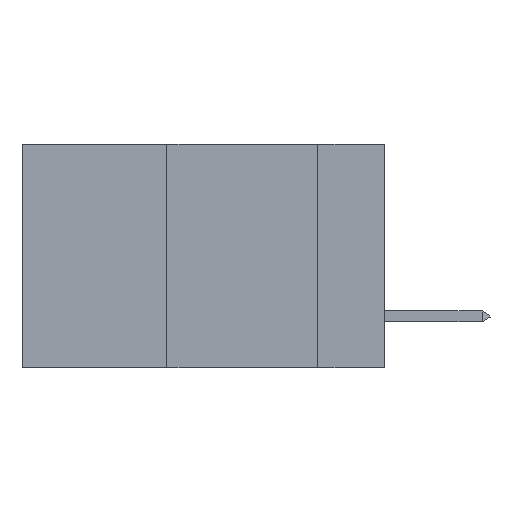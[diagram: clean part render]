
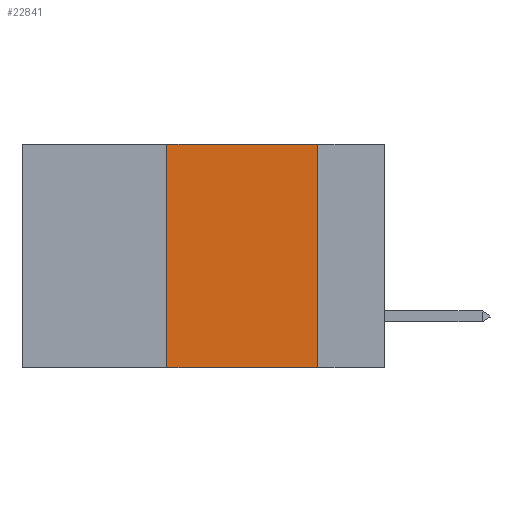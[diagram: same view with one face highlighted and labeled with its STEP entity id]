
A CAD part, left-side view. The second image highlights one B-rep face of the part: STEP entity #22841.
In plain terms, the highlighted planar face has unit normal (-1, 0, 0).
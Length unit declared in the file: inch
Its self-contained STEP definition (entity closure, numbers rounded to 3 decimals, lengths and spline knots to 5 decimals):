
#185 = CARTESIAN_POINT ( 'NONE',  ( 0., 0.6, 0. ) ) ;
#792 = CARTESIAN_POINT ( 'NONE',  ( 0., 0.36, 0. ) ) ;
#1187 = VERTEX_POINT ( 'NONE', #9490 ) ;
#1258 = VECTOR ( 'NONE', #18300, 39.37008 ) ;
#2068 = CARTESIAN_POINT ( 'NONE',  ( 0., 0.11, 0. ) ) ;
#2605 = DIRECTION ( 'NONE',  ( 0., 0., -1. ) ) ;
#3357 = ORIENTED_EDGE ( 'NONE', *, *, #15038, .T. ) ;
#3580 = ORIENTED_EDGE ( 'NONE', *, *, #14342, .F. ) ;
#4287 = DIRECTION ( 'NONE',  ( 1., 0., 0. ) ) ;
#4668 = CARTESIAN_POINT ( 'NONE',  ( 0., 0.11, -0.37 ) ) ;
#5337 = EDGE_CURVE ( 'NONE', #1187, #9684, #16919, .T. ) ;
#5397 = DIRECTION ( 'NONE',  ( 0., 0., -1. ) ) ;
#6260 = PLANE ( 'NONE',  #19993 ) ;
#6684 = EDGE_LOOP ( 'NONE', ( #13768, #13203, #3580, #3357 ) ) ;
#9490 = CARTESIAN_POINT ( 'NONE',  ( 0., 0.36, 0. ) ) ;
#9684 = VERTEX_POINT ( 'NONE', #2068 ) ;
#9961 = LINE ( 'NONE', #22613, #13605 ) ;
#10132 = CARTESIAN_POINT ( 'NONE',  ( 0., 0.6, 0. ) ) ;
#10228 = DIRECTION ( 'NONE',  ( 0., -1., 0. ) ) ;
#11106 = VECTOR ( 'NONE', #5397, 39.37008 ) ;
#12318 = FACE_OUTER_BOUND ( 'NONE', #6684, .T. ) ;
#13203 = ORIENTED_EDGE ( 'NONE', *, *, #5337, .F. ) ;
#13605 = VECTOR ( 'NONE', #10228, 39.37008 ) ;
#13768 = ORIENTED_EDGE ( 'NONE', *, *, #23247, .F. ) ;
#14205 = VECTOR ( 'NONE', #17595, 39.37008 ) ;
#14342 = EDGE_CURVE ( 'NONE', #24727, #1187, #15746, .T. ) ;
#15038 = EDGE_CURVE ( 'NONE', #24727, #21352, #9961, .T. ) ;
#15746 = LINE ( 'NONE', #792, #1258 ) ;
#15779 = CARTESIAN_POINT ( 'NONE',  ( 0., 0.36, -0.37 ) ) ;
#16919 = LINE ( 'NONE', #185, #14205 ) ;
#16937 = CARTESIAN_POINT ( 'NONE',  ( 0., 0.11, 0. ) ) ;
#17595 = DIRECTION ( 'NONE',  ( 0., -1., 0. ) ) ;
#18300 = DIRECTION ( 'NONE',  ( 0., 0., 1. ) ) ;
#19993 = AXIS2_PLACEMENT_3D ( 'NONE', #10132, #4287, #2605 ) ;
#21352 = VERTEX_POINT ( 'NONE', #4668 ) ;
#22612 = LINE ( 'NONE', #16937, #11106 ) ;
#22613 = CARTESIAN_POINT ( 'NONE',  ( 0., 0.6, -0.37 ) ) ;
#22841 = ADVANCED_FACE ( 'NONE', ( #12318 ), #6260, .F. ) ;
#23247 = EDGE_CURVE ( 'NONE', #9684, #21352, #22612, .T. ) ;
#24727 = VERTEX_POINT ( 'NONE', #15779 ) ;
